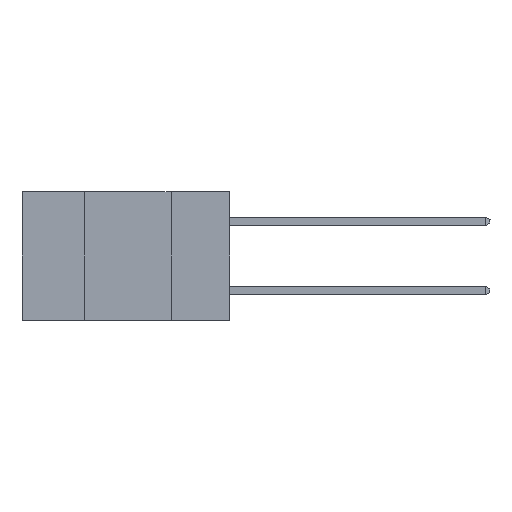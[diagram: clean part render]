
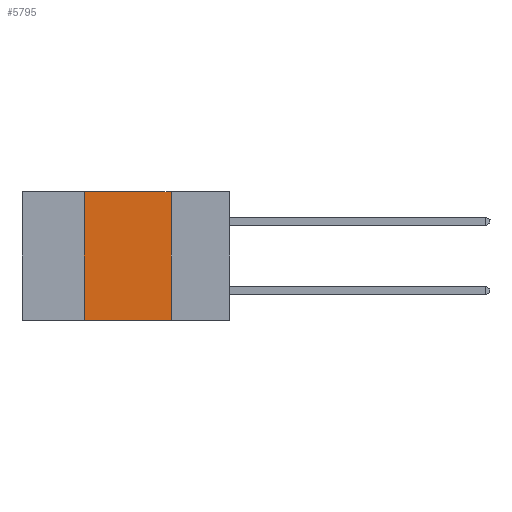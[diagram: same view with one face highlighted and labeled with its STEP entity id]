
A CAD part, left-side view. The second image highlights one B-rep face of the part: STEP entity #5795.
In plain terms, the highlighted planar face has unit normal (-1, 0, 0).
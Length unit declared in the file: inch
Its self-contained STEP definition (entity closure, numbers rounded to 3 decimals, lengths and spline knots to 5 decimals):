
#152 = CARTESIAN_POINT ( 'NONE',  ( 0., 0.17, 0. ) ) ;
#315 = CARTESIAN_POINT ( 'NONE',  ( 0., 0.6, -0.37 ) ) ;
#1122 = VECTOR ( 'NONE', #10032, 39.37008 ) ;
#1907 = LINE ( 'NONE', #3745, #2783 ) ;
#2565 = DIRECTION ( 'NONE',  ( 0., -1., 0. ) ) ;
#2715 = EDGE_CURVE ( 'NONE', #12792, #4561, #1907, .T. ) ;
#2783 = VECTOR ( 'NONE', #4683, 39.37008 ) ;
#3295 = VECTOR ( 'NONE', #2565, 39.37008 ) ;
#3733 = LINE ( 'NONE', #9539, #9741 ) ;
#3745 = CARTESIAN_POINT ( 'NONE',  ( 0., 0.17, 0. ) ) ;
#4366 = EDGE_LOOP ( 'NONE', ( #14557, #4876, #9339, #4907 ) ) ;
#4515 = VERTEX_POINT ( 'NONE', #6832 ) ;
#4561 = VERTEX_POINT ( 'NONE', #7837 ) ;
#4683 = DIRECTION ( 'NONE',  ( 0., 0., -1. ) ) ;
#4876 = ORIENTED_EDGE ( 'NONE', *, *, #13147, .F. ) ;
#4907 = ORIENTED_EDGE ( 'NONE', *, *, #12289, .T. ) ;
#5775 = LINE ( 'NONE', #315, #3295 ) ;
#5795 = ADVANCED_FACE ( 'NONE', ( #12813 ), #13848, .F. ) ;
#5989 = CARTESIAN_POINT ( 'NONE',  ( 0., 0.6, 0. ) ) ;
#6832 = CARTESIAN_POINT ( 'NONE',  ( 0., 0.42, 0. ) ) ;
#7051 = DIRECTION ( 'NONE',  ( 0., 0., -1. ) ) ;
#7754 = CARTESIAN_POINT ( 'NONE',  ( 0., 0.6, 0. ) ) ;
#7837 = CARTESIAN_POINT ( 'NONE',  ( 0., 0.17, -0.37 ) ) ;
#8117 = DIRECTION ( 'NONE',  ( 1., 0., 0. ) ) ;
#8878 = LINE ( 'NONE', #7754, #1122 ) ;
#9339 = ORIENTED_EDGE ( 'NONE', *, *, #9975, .F. ) ;
#9539 = CARTESIAN_POINT ( 'NONE',  ( 0., 0.42, 0. ) ) ;
#9741 = VECTOR ( 'NONE', #10628, 39.37008 ) ;
#9975 = EDGE_CURVE ( 'NONE', #11779, #4515, #3733, .T. ) ;
#10032 = DIRECTION ( 'NONE',  ( 0., -1., 0. ) ) ;
#10628 = DIRECTION ( 'NONE',  ( 0., 0., 1. ) ) ;
#11376 = CARTESIAN_POINT ( 'NONE',  ( 0., 0.42, -0.37 ) ) ;
#11779 = VERTEX_POINT ( 'NONE', #11376 ) ;
#12289 = EDGE_CURVE ( 'NONE', #11779, #4561, #5775, .T. ) ;
#12792 = VERTEX_POINT ( 'NONE', #152 ) ;
#12813 = FACE_OUTER_BOUND ( 'NONE', #4366, .T. ) ;
#12948 = AXIS2_PLACEMENT_3D ( 'NONE', #5989, #8117, #7051 ) ;
#13147 = EDGE_CURVE ( 'NONE', #4515, #12792, #8878, .T. ) ;
#13848 = PLANE ( 'NONE',  #12948 ) ;
#14557 = ORIENTED_EDGE ( 'NONE', *, *, #2715, .F. ) ;
